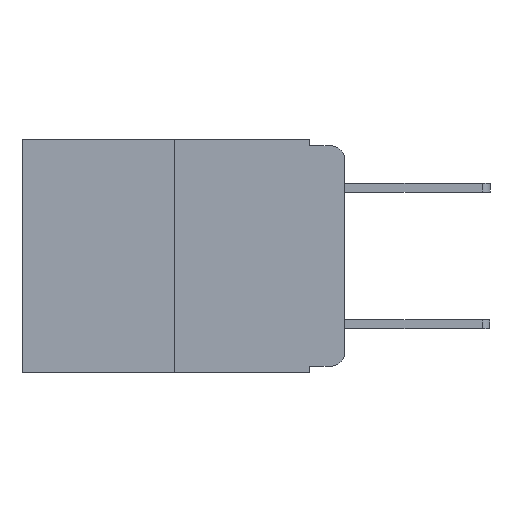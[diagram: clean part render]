
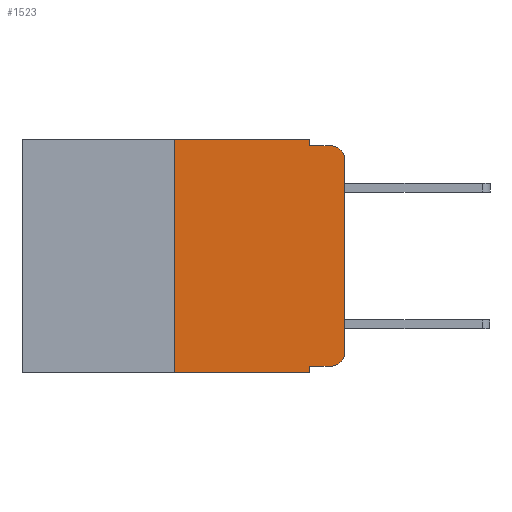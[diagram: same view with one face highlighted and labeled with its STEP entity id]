
A CAD part, left-side view. The second image highlights one B-rep face of the part: STEP entity #1523.
In plain terms, the highlighted planar face has unit normal (-1, 0, 0).
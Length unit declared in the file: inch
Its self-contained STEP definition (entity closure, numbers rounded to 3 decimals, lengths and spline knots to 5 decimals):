
#579 = ORIENTED_EDGE ( 'NONE', *, *, #8851, .T. ) ;
#1354 = ORIENTED_EDGE ( 'NONE', *, *, #7497, .T. ) ;
#1397 = AXIS2_PLACEMENT_3D ( 'NONE', #7887, #17551, #9342 ) ;
#1523 = ADVANCED_FACE ( 'NONE', ( #13636 ), #16486, .F. ) ;
#1657 = ORIENTED_EDGE ( 'NONE', *, *, #15464, .F. ) ;
#2229 = ORIENTED_EDGE ( 'NONE', *, *, #13299, .F. ) ;
#2392 = ORIENTED_EDGE ( 'NONE', *, *, #18571, .F. ) ;
#2436 = ORIENTED_EDGE ( 'NONE', *, *, #9234, .F. ) ;
#2729 = EDGE_CURVE ( 'NONE', #4032, #17096, #8962, .T. ) ;
#2732 = VECTOR ( 'NONE', #15570, 39.37008 ) ;
#2761 = ORIENTED_EDGE ( 'NONE', *, *, #14754, .T. ) ;
#2876 = ORIENTED_EDGE ( 'NONE', *, *, #2729, .F. ) ;
#2893 = CARTESIAN_POINT ( 'NONE',  ( 0., 0.051, -0.333 ) ) ;
#2907 = ORIENTED_EDGE ( 'NONE', *, *, #12603, .T. ) ;
#3023 = LINE ( 'NONE', #15536, #7594 ) ;
#3167 = ORIENTED_EDGE ( 'NONE', *, *, #9640, .T. ) ;
#3180 = VERTEX_POINT ( 'NONE', #10622 ) ;
#3482 = VERTEX_POINT ( 'NONE', #14875 ) ;
#3930 = VECTOR ( 'NONE', #8231, 39.37008 ) ;
#3949 = CARTESIAN_POINT ( 'NONE',  ( 0., 0.051, 0. ) ) ;
#3951 = VERTEX_POINT ( 'NONE', #16051 ) ;
#4032 = VERTEX_POINT ( 'NONE', #2893 ) ;
#4162 = CARTESIAN_POINT ( 'NONE',  ( 0., 0.051, 0. ) ) ;
#4643 = CARTESIAN_POINT ( 'NONE',  ( 0., 0.473, -0.343 ) ) ;
#5013 = CARTESIAN_POINT ( 'NONE',  ( 0., 0.051, -0.01 ) ) ;
#5702 = VECTOR ( 'NONE', #10857, 39.37008 ) ;
#5806 = LINE ( 'NONE', #14822, #10141 ) ;
#5976 = DIRECTION ( 'NONE',  ( 0., 0., 1. ) ) ;
#6203 = LINE ( 'NONE', #5013, #5702 ) ;
#6407 = DIRECTION ( 'NONE',  ( 0., -1., 0. ) ) ;
#6961 = CARTESIAN_POINT ( 'NONE',  ( 0., 0.051, -0.343 ) ) ;
#7171 = DIRECTION ( 'NONE',  ( 0., -1., 0. ) ) ;
#7398 = CARTESIAN_POINT ( 'NONE',  ( 0., 0., 0. ) ) ;
#7497 = EDGE_CURVE ( 'NONE', #3951, #3482, #10125, .T. ) ;
#7551 = CARTESIAN_POINT ( 'NONE',  ( 0., 0.051, -0.01 ) ) ;
#7594 = VECTOR ( 'NONE', #7171, 39.37008 ) ;
#7887 = CARTESIAN_POINT ( 'NONE',  ( 0., 0.02, -0.03 ) ) ;
#7965 = LINE ( 'NONE', #12383, #3930 ) ;
#8231 = DIRECTION ( 'NONE',  ( 0., 0., 1. ) ) ;
#8611 = VERTEX_POINT ( 'NONE', #14073 ) ;
#8693 = DIRECTION ( 'NONE',  ( 0., 0., -1. ) ) ;
#8851 = EDGE_CURVE ( 'NONE', #10446, #3951, #17691, .T. ) ;
#8944 = CARTESIAN_POINT ( 'NONE',  ( 0., 0.02, -0.313 ) ) ;
#8962 = LINE ( 'NONE', #15575, #15850 ) ;
#9234 = EDGE_CURVE ( 'NONE', #14156, #8611, #7965, .T. ) ;
#9342 = DIRECTION ( 'NONE',  ( 0., 0., -1. ) ) ;
#9392 = AXIS2_PLACEMENT_3D ( 'NONE', #8944, #18508, #10341 ) ;
#9640 = EDGE_CURVE ( 'NONE', #3180, #10446, #12056, .T. ) ;
#10125 = CIRCLE ( 'NONE', #1397, 0.02 ) ;
#10141 = VECTOR ( 'NONE', #6407, 39.37008 ) ;
#10290 = LINE ( 'NONE', #4643, #17562 ) ;
#10341 = DIRECTION ( 'NONE',  ( 0., 0., -1. ) ) ;
#10446 = VERTEX_POINT ( 'NONE', #16055 ) ;
#10622 = CARTESIAN_POINT ( 'NONE',  ( 0., 0.02, -0.333 ) ) ;
#10832 = EDGE_LOOP ( 'NONE', ( #579, #1354, #1657, #2229, #2392, #2436, #2761, #2876, #2907, #3167 ) ) ;
#10857 = DIRECTION ( 'NONE',  ( 0., -1., 0. ) ) ;
#12056 = CIRCLE ( 'NONE', #9392, 0.02 ) ;
#12113 = CARTESIAN_POINT ( 'NONE',  ( 0., 0.25, -0.343 ) ) ;
#12383 = CARTESIAN_POINT ( 'NONE',  ( 0., 0.25, 0. ) ) ;
#12603 = EDGE_CURVE ( 'NONE', #4032, #3180, #3023, .T. ) ;
#12744 = VERTEX_POINT ( 'NONE', #7551 ) ;
#13299 = EDGE_CURVE ( 'NONE', #18812, #12744, #14794, .T. ) ;
#13636 = FACE_OUTER_BOUND ( 'NONE', #10832, .T. ) ;
#14073 = CARTESIAN_POINT ( 'NONE',  ( 0., 0.25, 0. ) ) ;
#14083 = VECTOR ( 'NONE', #5976, 39.37008 ) ;
#14156 = VERTEX_POINT ( 'NONE', #12113 ) ;
#14754 = EDGE_CURVE ( 'NONE', #14156, #17096, #10290, .T. ) ;
#14794 = LINE ( 'NONE', #4162, #2732 ) ;
#14822 = CARTESIAN_POINT ( 'NONE',  ( 0., 0.473, 0. ) ) ;
#14875 = CARTESIAN_POINT ( 'NONE',  ( 0., 0.02, -0.01 ) ) ;
#15129 = CARTESIAN_POINT ( 'NONE',  ( 0., 0.473, 0. ) ) ;
#15464 = EDGE_CURVE ( 'NONE', #12744, #3482, #6203, .T. ) ;
#15536 = CARTESIAN_POINT ( 'NONE',  ( 0., 0.051, -0.333 ) ) ;
#15570 = DIRECTION ( 'NONE',  ( 0., 0., -1. ) ) ;
#15575 = CARTESIAN_POINT ( 'NONE',  ( 0., 0.051, 0. ) ) ;
#15850 = VECTOR ( 'NONE', #8693, 39.37008 ) ;
#15970 = DIRECTION ( 'NONE',  ( 0., 0., -1. ) ) ;
#16051 = CARTESIAN_POINT ( 'NONE',  ( 0., 0., -0.03 ) ) ;
#16055 = CARTESIAN_POINT ( 'NONE',  ( 0., 0., -0.313 ) ) ;
#16485 = AXIS2_PLACEMENT_3D ( 'NONE', #15129, #16857, #15970 ) ;
#16486 = PLANE ( 'NONE',  #16485 ) ;
#16857 = DIRECTION ( 'NONE',  ( 1., 0., 0. ) ) ;
#17096 = VERTEX_POINT ( 'NONE', #6961 ) ;
#17340 = DIRECTION ( 'NONE',  ( 0., -1., 0. ) ) ;
#17551 = DIRECTION ( 'NONE',  ( -1., 0., 0. ) ) ;
#17562 = VECTOR ( 'NONE', #17340, 39.37008 ) ;
#17691 = LINE ( 'NONE', #7398, #14083 ) ;
#18508 = DIRECTION ( 'NONE',  ( -1., 0., 0. ) ) ;
#18571 = EDGE_CURVE ( 'NONE', #8611, #18812, #5806, .T. ) ;
#18812 = VERTEX_POINT ( 'NONE', #3949 ) ;
